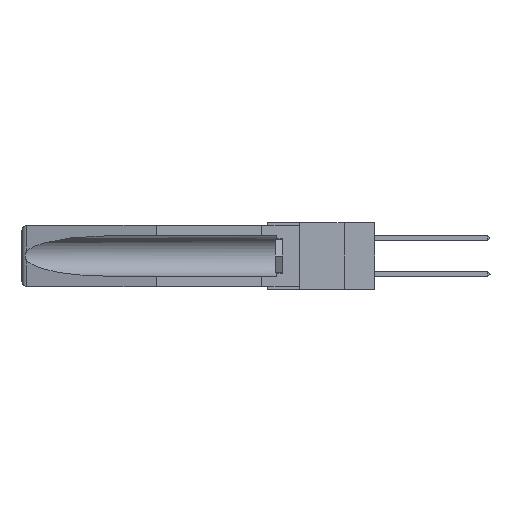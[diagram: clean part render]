
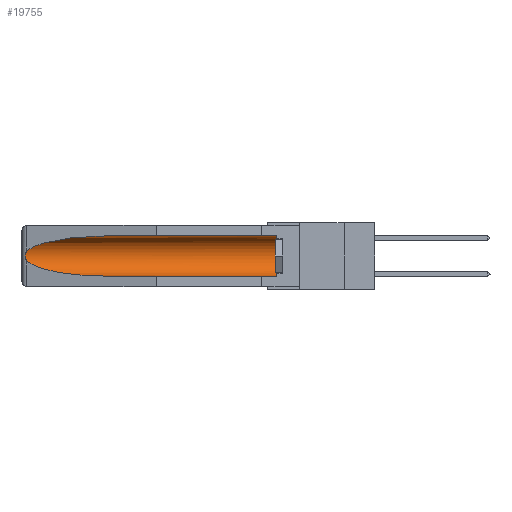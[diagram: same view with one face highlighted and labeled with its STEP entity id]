
A CAD part, left-side view. The second image highlights one B-rep face of the part: STEP entity #19755.
In plain terms, the highlighted cylindrical face has radius 2.857 mm (diameter 5.715 mm), a partial arc.
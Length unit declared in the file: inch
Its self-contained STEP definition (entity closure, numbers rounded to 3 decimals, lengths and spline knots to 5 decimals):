
#34 = CARTESIAN_POINT ( 'NONE',  ( 0.26654, 1.53092, -0.15636 ) ) ;
#53 = EDGE_CURVE ( 'NONE', #26544, #22998, #20064, .T. ) ;
#108 = ORIENTED_EDGE ( 'NONE', *, *, #1605, .F. ) ;
#130 = CARTESIAN_POINT ( 'NONE',  ( 0.26597, 1.52961, -0.15275 ) ) ;
#1605 = EDGE_CURVE ( 'NONE', #19020, #22998, #12759, .T. ) ;
#2747 = ORIENTED_EDGE ( 'NONE', *, *, #13868, .T. ) ;
#2951 = CARTESIAN_POINT ( 'NONE',  ( 0.21114, 1.30732, -0.059 ) ) ;
#3071 = DIRECTION ( 'NONE',  ( 0., -1., 0. ) ) ;
#3487 = VERTEX_POINT ( 'NONE', #16971 ) ;
#3524 = AXIS2_PLACEMENT_3D ( 'NONE', #6985, #14037, #23627 ) ;
#3580 = VECTOR ( 'NONE', #27917, 39.37008 ) ;
#4121 = CARTESIAN_POINT ( 'NONE',  ( 0.155, 1.07973, -0.284 ) ) ;
#6248 = FACE_OUTER_BOUND ( 'NONE', #30467, .T. ) ;
#6985 = CARTESIAN_POINT ( 'NONE',  ( 0.155, -0.30754, -0.1715 ) ) ;
#7194 = CARTESIAN_POINT ( 'NONE',  ( 0.2675, 1.53308, -0.17534 ) ) ;
#7933 = CARTESIAN_POINT ( 'NONE',  ( 0.26537, 1.52718, -0.14972 ) ) ;
#8719 = CARTESIAN_POINT ( 'NONE',  ( 0.21114, 1.30732, -0.284 ) ) ;
#9530 = EDGE_CURVE ( 'NONE', #3487, #19450, #18400, .T. ) ;
#9550 = CARTESIAN_POINT ( 'NONE',  ( 0.26537, 1.52718, -0.14972 ) ) ;
#9648 = CARTESIAN_POINT ( 'NONE',  ( 0.2675, 1.53308, -0.16763 ) ) ;
#10236 = DIRECTION ( 'NONE',  ( 0., 1., 0. ) ) ;
#10977 = CARTESIAN_POINT ( 'NONE',  ( 0.155, 1.07973, -0.284 ) ) ;
#12759 = LINE ( 'NONE', #17409, #22415 ) ;
#13173 = CARTESIAN_POINT ( 'NONE',  ( 0.25451, 1.48313, -0.24835 ) ) ;
#13639 = CARTESIAN_POINT ( 'NONE',  ( 0.26537, 1.52718, -0.14972 ) ) ;
#13868 = EDGE_CURVE ( 'NONE', #15926, #26544, #27061, .T. ) ;
#14037 = DIRECTION ( 'NONE',  ( 0., 1., 0. ) ) ;
#14042 = CARTESIAN_POINT ( 'NONE',  ( 0.2673, 1.5327, -0.16383 ) ) ;
#14149 = CARTESIAN_POINT ( 'NONE',  ( 0.26597, 1.5296, -0.19026 ) ) ;
#15926 = VERTEX_POINT ( 'NONE', #13639 ) ;
#16971 = CARTESIAN_POINT ( 'NONE',  ( 0.155, 0.126, -0.059 ) ) ;
#17409 = CARTESIAN_POINT ( 'NONE',  ( 0.155, -0.30754, -0.284 ) ) ;
#18063 = AXIS2_PLACEMENT_3D ( 'NONE', #24179, #3071, #29124 ) ;
#18147 = ORIENTED_EDGE ( 'NONE', *, *, #9530, .T. ) ;
#18400 = LINE ( 'NONE', #23666, #3580 ) ;
#18784 = ORIENTED_EDGE ( 'NONE', *, *, #25676, .T. ) ;
#18895 = CARTESIAN_POINT ( 'NONE',  ( 0.2673, 1.53269, -0.17917 ) ) ;
#19020 = VERTEX_POINT ( 'NONE', #21326 ) ;
#19450 = VERTEX_POINT ( 'NONE', #22239 ) ;
#19512 = CIRCLE ( 'NONE', #18063, 0.1125 ) ;
#19606 = ORIENTED_EDGE ( 'NONE', *, *, #53, .T. ) ;
#19755 = ADVANCED_FACE ( 'NONE', ( #6248 ), #20660, .F. ) ;
#19980 = ORIENTED_EDGE ( 'NONE', *, *, #29134, .T. ) ;
#20064 =( BOUNDED_CURVE ( )  B_SPLINE_CURVE ( 3, ( #24961, #13173, #8719, #10977 ),
 .UNSPECIFIED., .F., .F. ) 
 B_SPLINE_CURVE_WITH_KNOTS ( ( 4, 4 ),
 ( 0.1948, 1.5708 ),
 .UNSPECIFIED. ) 
 CURVE ( )  GEOMETRIC_REPRESENTATION_ITEM ( )  RATIONAL_B_SPLINE_CURVE ( ( 1., 0.848, 0.848, 1. ) ) 
 REPRESENTATION_ITEM ( '' )  );
#20660 = CYLINDRICAL_SURFACE ( 'NONE', #3524, 0.1125 ) ;
#21326 = CARTESIAN_POINT ( 'NONE',  ( 0.155, 0.126, -0.284 ) ) ;
#22239 = CARTESIAN_POINT ( 'NONE',  ( 0.155, 1.07973, -0.059 ) ) ;
#22415 = VECTOR ( 'NONE', #10236, 39.37008 ) ;
#22998 = VERTEX_POINT ( 'NONE', #4121 ) ;
#23627 = DIRECTION ( 'NONE',  ( 0., 0., 1. ) ) ;
#23666 = CARTESIAN_POINT ( 'NONE',  ( 0.155, -0.30754, -0.059 ) ) ;
#24179 = CARTESIAN_POINT ( 'NONE',  ( 0.155, 0.126, -0.1715 ) ) ;
#24363 = CARTESIAN_POINT ( 'NONE',  ( 0.25451, 1.48313, -0.09465 ) ) ;
#24961 = CARTESIAN_POINT ( 'NONE',  ( 0.26537, 1.52718, -0.19328 ) ) ;
#25676 = EDGE_CURVE ( 'NONE', #19450, #15926, #30288, .T. ) ;
#26125 = CARTESIAN_POINT ( 'NONE',  ( 0.26655, 1.53094, -0.18657 ) ) ;
#26544 = VERTEX_POINT ( 'NONE', #27322 ) ;
#27061 = B_SPLINE_CURVE_WITH_KNOTS ( 'NONE', 3,
 ( #9550, #130, #34, #14042, #9648, #7194, #18895, #26125, #14149, #30572 ),
 .UNSPECIFIED., .F., .F.,
 ( 4, 2, 2, 2, 4 ),
 ( 0., 0.00029, 0.00058, 0.00087, 0.00117 ),
 .UNSPECIFIED. ) ;
#27322 = CARTESIAN_POINT ( 'NONE',  ( 0.26537, 1.52718, -0.19328 ) ) ;
#27917 = DIRECTION ( 'NONE',  ( 0., 1., 0. ) ) ;
#28798 = CARTESIAN_POINT ( 'NONE',  ( 0.155, 1.07973, -0.059 ) ) ;
#29124 = DIRECTION ( 'NONE',  ( 0., 0., 1. ) ) ;
#29134 = EDGE_CURVE ( 'NONE', #19020, #3487, #19512, .T. ) ;
#30288 =( BOUNDED_CURVE ( )  B_SPLINE_CURVE ( 3, ( #28798, #2951, #24363, #7933 ),
 .UNSPECIFIED., .F., .F. ) 
 B_SPLINE_CURVE_WITH_KNOTS ( ( 4, 4 ),
 ( 4.71239, 6.08839 ),
 .UNSPECIFIED. ) 
 CURVE ( )  GEOMETRIC_REPRESENTATION_ITEM ( )  RATIONAL_B_SPLINE_CURVE ( ( 1., 0.848, 0.848, 1. ) ) 
 REPRESENTATION_ITEM ( '' )  );
#30467 = EDGE_LOOP ( 'NONE', ( #18784, #2747, #19606, #108, #19980, #18147 ) ) ;
#30572 = CARTESIAN_POINT ( 'NONE',  ( 0.26537, 1.52718, -0.19328 ) ) ;
